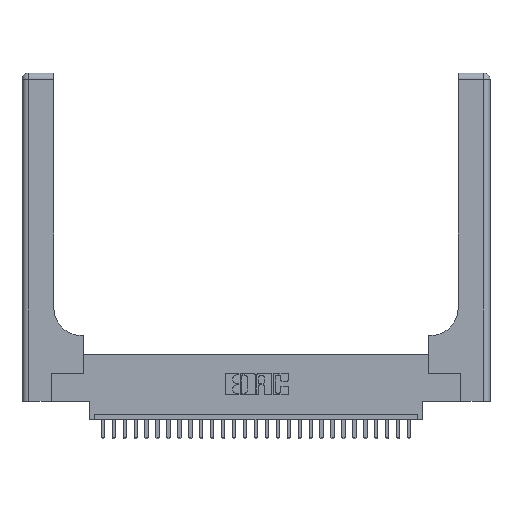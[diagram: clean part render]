
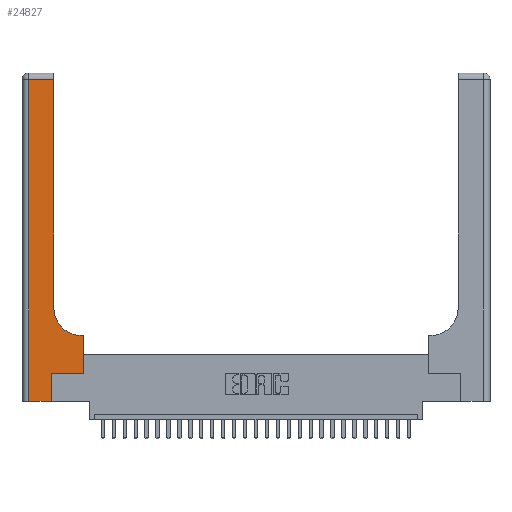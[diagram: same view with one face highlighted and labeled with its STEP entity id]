
A CAD part, top view. The second image highlights one B-rep face of the part: STEP entity #24827.
In plain terms, the highlighted planar face has unit normal (0, 0, 1).
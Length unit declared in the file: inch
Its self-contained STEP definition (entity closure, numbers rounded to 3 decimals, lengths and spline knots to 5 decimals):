
#715 = DIRECTION ( 'NONE',  ( 0., 1., 0. ) ) ;
#792 = VECTOR ( 'NONE', #7872, 39.37008 ) ;
#817 = CARTESIAN_POINT ( 'NONE',  ( 0.5585, 0.25, 0.37 ) ) ;
#847 = ORIENTED_EDGE ( 'NONE', *, *, #8514, .T. ) ;
#1099 = CARTESIAN_POINT ( 'NONE',  ( 0., 2.94, 0.37 ) ) ;
#1779 = DIRECTION ( 'NONE',  ( 0., -1., 0. ) ) ;
#2060 = VERTEX_POINT ( 'NONE', #9365 ) ;
#2222 = LINE ( 'NONE', #1099, #792 ) ;
#2325 = CARTESIAN_POINT ( 'NONE',  ( 0.5415, 0.85, 0.37 ) ) ;
#2418 = LINE ( 'NONE', #5247, #4502 ) ;
#2797 = AXIS2_PLACEMENT_3D ( 'NONE', #2325, #8783, #24487 ) ;
#3069 = EDGE_LOOP ( 'NONE', ( #4889, #20120, #6258, #8380, #17634, #9811, #847, #23797, #22830 ) ) ;
#3916 = DIRECTION ( 'NONE',  ( 0., 0., -1. ) ) ;
#4046 = CARTESIAN_POINT ( 'NONE',  ( 0.2915, 0.6, 0.37 ) ) ;
#4120 = LINE ( 'NONE', #817, #17440 ) ;
#4502 = VECTOR ( 'NONE', #9446, 39.37008 ) ;
#4632 = VERTEX_POINT ( 'NONE', #28194 ) ;
#4889 = ORIENTED_EDGE ( 'NONE', *, *, #16126, .T. ) ;
#5247 = CARTESIAN_POINT ( 'NONE',  ( 0., 0., 0.37 ) ) ;
#6050 = LINE ( 'NONE', #16870, #10256 ) ;
#6258 = ORIENTED_EDGE ( 'NONE', *, *, #12459, .T. ) ;
#6670 = VERTEX_POINT ( 'NONE', #14602 ) ;
#7070 = CARTESIAN_POINT ( 'NONE',  ( 0.2915, 0.85, 0.37 ) ) ;
#7872 = DIRECTION ( 'NONE',  ( -1., 0., 0. ) ) ;
#8201 = CARTESIAN_POINT ( 'NONE',  ( 0.269, 0., 0.37 ) ) ;
#8380 = ORIENTED_EDGE ( 'NONE', *, *, #17836, .T. ) ;
#8504 = LINE ( 'NONE', #26678, #17610 ) ;
#8514 = EDGE_CURVE ( 'NONE', #4632, #20159, #4120, .T. ) ;
#8704 = LINE ( 'NONE', #24138, #25160 ) ;
#8783 = DIRECTION ( 'NONE',  ( 0., 0., -1. ) ) ;
#9365 = CARTESIAN_POINT ( 'NONE',  ( 0.269, 0.25, 0.37 ) ) ;
#9446 = DIRECTION ( 'NONE',  ( 1., 0., 0. ) ) ;
#9811 = ORIENTED_EDGE ( 'NONE', *, *, #11218, .T. ) ;
#10256 = VECTOR ( 'NONE', #20002, 39.37008 ) ;
#10350 = PLANE ( 'NONE',  #25821 ) ;
#10590 = CARTESIAN_POINT ( 'NONE',  ( 0.2915, 2.94, 0.37 ) ) ;
#10747 = DIRECTION ( 'NONE',  ( -1., 0., 0. ) ) ;
#11164 = EDGE_CURVE ( 'NONE', #24228, #6670, #2222, .T. ) ;
#11218 = EDGE_CURVE ( 'NONE', #2060, #4632, #6050, .T. ) ;
#12160 = VERTEX_POINT ( 'NONE', #23068 ) ;
#12459 = EDGE_CURVE ( 'NONE', #6670, #14755, #8704, .T. ) ;
#12460 = CARTESIAN_POINT ( 'NONE',  ( 0.269, 0., 0.37 ) ) ;
#12551 = EDGE_CURVE ( 'NONE', #20159, #12160, #17206, .T. ) ;
#13294 = FACE_OUTER_BOUND ( 'NONE', #3069, .T. ) ;
#13517 = CARTESIAN_POINT ( 'NONE',  ( 0.06, 0., 0.37 ) ) ;
#14129 = CARTESIAN_POINT ( 'NONE',  ( 0.5585, 0.6, 0.37 ) ) ;
#14602 = CARTESIAN_POINT ( 'NONE',  ( 0.06, 2.94, 0.37 ) ) ;
#14755 = VERTEX_POINT ( 'NONE', #13517 ) ;
#16126 = EDGE_CURVE ( 'NONE', #21148, #24228, #8504, .T. ) ;
#16598 = DIRECTION ( 'NONE',  ( 0., 1., 0. ) ) ;
#16870 = CARTESIAN_POINT ( 'NONE',  ( 0.269, 0.25, 0.37 ) ) ;
#17206 = LINE ( 'NONE', #4046, #24927 ) ;
#17440 = VECTOR ( 'NONE', #715, 39.37008 ) ;
#17610 = VECTOR ( 'NONE', #17645, 39.37008 ) ;
#17634 = ORIENTED_EDGE ( 'NONE', *, *, #22967, .T. ) ;
#17645 = DIRECTION ( 'NONE',  ( 0., 1., 0. ) ) ;
#17658 = VECTOR ( 'NONE', #16598, 39.37008 ) ;
#17836 = EDGE_CURVE ( 'NONE', #14755, #22584, #2418, .T. ) ;
#18155 = EDGE_CURVE ( 'NONE', #12160, #21148, #21664, .T. ) ;
#20002 = DIRECTION ( 'NONE',  ( 1., 0., 0. ) ) ;
#20120 = ORIENTED_EDGE ( 'NONE', *, *, #11164, .T. ) ;
#20159 = VERTEX_POINT ( 'NONE', #14129 ) ;
#21148 = VERTEX_POINT ( 'NONE', #7070 ) ;
#21664 = CIRCLE ( 'NONE', #2797, 0.25 ) ;
#21826 = CARTESIAN_POINT ( 'NONE',  ( 0., 3., 0.37 ) ) ;
#22584 = VERTEX_POINT ( 'NONE', #8201 ) ;
#22830 = ORIENTED_EDGE ( 'NONE', *, *, #18155, .T. ) ;
#22967 = EDGE_CURVE ( 'NONE', #22584, #2060, #28137, .T. ) ;
#23068 = CARTESIAN_POINT ( 'NONE',  ( 0.5415, 0.6, 0.37 ) ) ;
#23797 = ORIENTED_EDGE ( 'NONE', *, *, #12551, .T. ) ;
#24138 = CARTESIAN_POINT ( 'NONE',  ( 0.06, 3., 0.37 ) ) ;
#24228 = VERTEX_POINT ( 'NONE', #10590 ) ;
#24487 = DIRECTION ( 'NONE',  ( 1., 0., 0. ) ) ;
#24827 = ADVANCED_FACE ( 'NONE', ( #13294 ), #10350, .F. ) ;
#24927 = VECTOR ( 'NONE', #28048, 39.37008 ) ;
#25160 = VECTOR ( 'NONE', #1779, 39.37008 ) ;
#25821 = AXIS2_PLACEMENT_3D ( 'NONE', #21826, #3916, #10747 ) ;
#26678 = CARTESIAN_POINT ( 'NONE',  ( 0.2915, 3., 0.37 ) ) ;
#28048 = DIRECTION ( 'NONE',  ( -1., 0., 0. ) ) ;
#28137 = LINE ( 'NONE', #12460, #17658 ) ;
#28194 = CARTESIAN_POINT ( 'NONE',  ( 0.5585, 0.25, 0.37 ) ) ;
